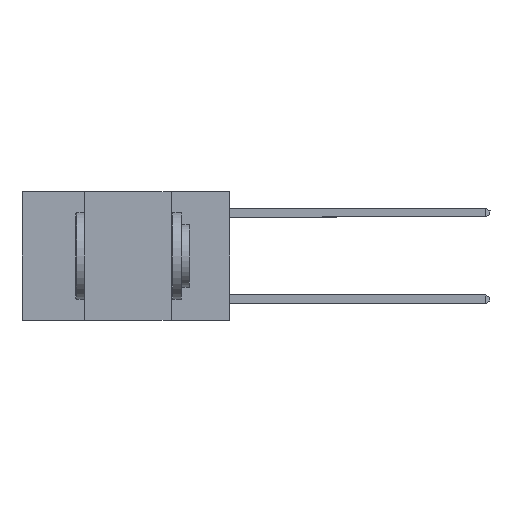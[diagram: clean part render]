
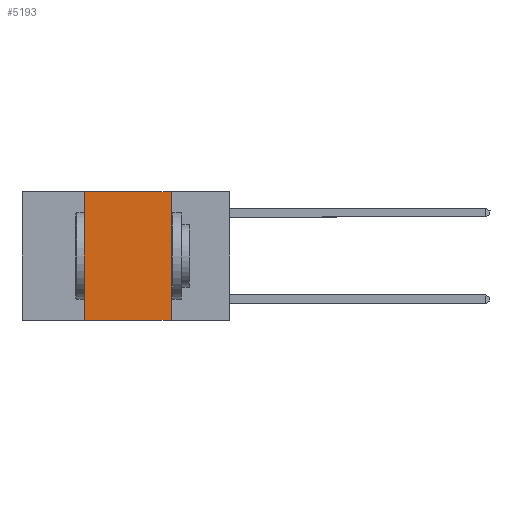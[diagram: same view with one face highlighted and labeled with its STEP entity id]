
A CAD part, left-side view. The second image highlights one B-rep face of the part: STEP entity #5193.
In plain terms, the highlighted planar face has unit normal (-1, 0, 0).
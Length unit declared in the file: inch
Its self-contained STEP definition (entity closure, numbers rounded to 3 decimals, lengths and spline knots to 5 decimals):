
#257 = CARTESIAN_POINT ( 'NONE',  ( 0., 0.17, 0. ) ) ;
#297 = CARTESIAN_POINT ( 'NONE',  ( 0., 0.42, 0. ) ) ;
#910 = DIRECTION ( 'NONE',  ( 0., 0., -1. ) ) ;
#1017 = VERTEX_POINT ( 'NONE', #6456 ) ;
#1076 = DIRECTION ( 'NONE',  ( 0., -1., 0. ) ) ;
#1544 = CARTESIAN_POINT ( 'NONE',  ( 0., 0.42, -0.37 ) ) ;
#2044 = CARTESIAN_POINT ( 'NONE',  ( 0., 0.17, 0. ) ) ;
#2223 = LINE ( 'NONE', #2044, #4061 ) ;
#2667 = EDGE_CURVE ( 'NONE', #3924, #6423, #2223, .T. ) ;
#3742 = LINE ( 'NONE', #3837, #9300 ) ;
#3757 = AXIS2_PLACEMENT_3D ( 'NONE', #8598, #5592, #910 ) ;
#3823 = CARTESIAN_POINT ( 'NONE',  ( 0., 0.17, -0.37 ) ) ;
#3837 = CARTESIAN_POINT ( 'NONE',  ( 0., 0.6, -0.37 ) ) ;
#3878 = VECTOR ( 'NONE', #9494, 39.37008 ) ;
#3924 = VERTEX_POINT ( 'NONE', #257 ) ;
#4061 = VECTOR ( 'NONE', #6657, 39.37008 ) ;
#4334 = LINE ( 'NONE', #5744, #6171 ) ;
#5193 = ADVANCED_FACE ( 'NONE', ( #9566 ), #7060, .F. ) ;
#5592 = DIRECTION ( 'NONE',  ( 1., 0., 0. ) ) ;
#5699 = EDGE_CURVE ( 'NONE', #1017, #3924, #4334, .T. ) ;
#5744 = CARTESIAN_POINT ( 'NONE',  ( 0., 0.6, 0. ) ) ;
#5917 = LINE ( 'NONE', #297, #3878 ) ;
#6171 = VECTOR ( 'NONE', #1076, 39.37008 ) ;
#6423 = VERTEX_POINT ( 'NONE', #3823 ) ;
#6456 = CARTESIAN_POINT ( 'NONE',  ( 0., 0.42, 0. ) ) ;
#6657 = DIRECTION ( 'NONE',  ( 0., 0., -1. ) ) ;
#6687 = EDGE_CURVE ( 'NONE', #7227, #1017, #5917, .T. ) ;
#7060 = PLANE ( 'NONE',  #3757 ) ;
#7227 = VERTEX_POINT ( 'NONE', #1544 ) ;
#7454 = EDGE_LOOP ( 'NONE', ( #7972, #7978, #8240, #9339 ) ) ;
#7783 = EDGE_CURVE ( 'NONE', #7227, #6423, #3742, .T. ) ;
#7972 = ORIENTED_EDGE ( 'NONE', *, *, #2667, .F. ) ;
#7978 = ORIENTED_EDGE ( 'NONE', *, *, #5699, .F. ) ;
#8240 = ORIENTED_EDGE ( 'NONE', *, *, #6687, .F. ) ;
#8598 = CARTESIAN_POINT ( 'NONE',  ( 0., 0.6, 0. ) ) ;
#9094 = DIRECTION ( 'NONE',  ( 0., -1., 0. ) ) ;
#9300 = VECTOR ( 'NONE', #9094, 39.37008 ) ;
#9339 = ORIENTED_EDGE ( 'NONE', *, *, #7783, .T. ) ;
#9494 = DIRECTION ( 'NONE',  ( 0., 0., 1. ) ) ;
#9566 = FACE_OUTER_BOUND ( 'NONE', #7454, .T. ) ;
